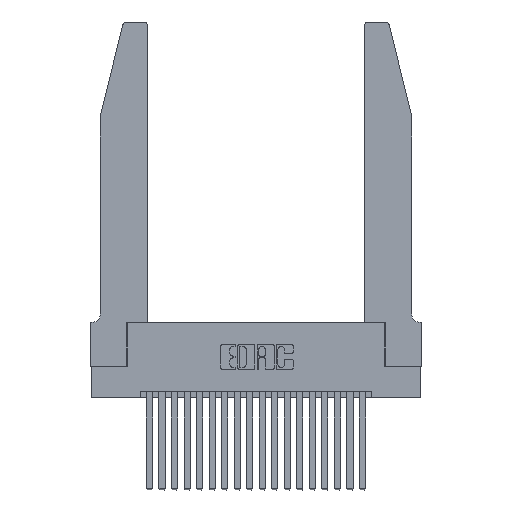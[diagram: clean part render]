
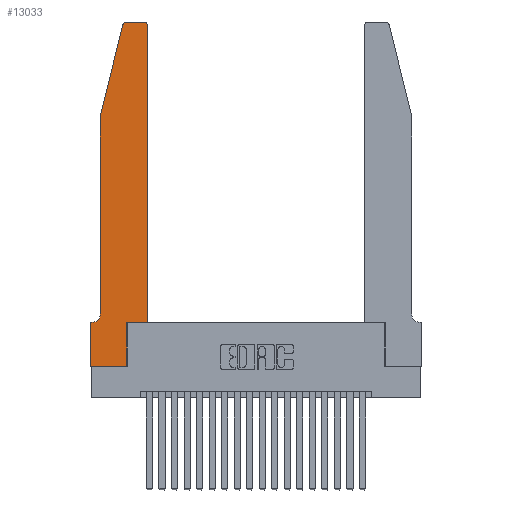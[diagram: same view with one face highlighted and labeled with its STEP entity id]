
A CAD part, top view. The second image highlights one B-rep face of the part: STEP entity #13033.
In plain terms, the highlighted planar face has unit normal (0, 0, 1).
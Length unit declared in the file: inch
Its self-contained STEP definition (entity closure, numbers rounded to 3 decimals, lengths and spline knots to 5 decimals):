
#79 = VERTEX_POINT ( 'NONE', #5755 ) ;
#144 = VERTEX_POINT ( 'NONE', #3099 ) ;
#146 = AXIS2_PLACEMENT_3D ( 'NONE', #11177, #937, #12860 ) ;
#159 = CARTESIAN_POINT ( 'NONE',  ( 0.0755, 2., 0.37 ) ) ;
#636 = EDGE_CURVE ( 'NONE', #144, #15574, #2656, .T. ) ;
#766 = CARTESIAN_POINT ( 'NONE',  ( 0.2865, 0.35, 0.37 ) ) ;
#859 = VECTOR ( 'NONE', #21269, 39.37008 ) ;
#937 = DIRECTION ( 'NONE',  ( 0., 0., -1. ) ) ;
#1041 = VERTEX_POINT ( 'NONE', #2652 ) ;
#1307 = EDGE_CURVE ( 'NONE', #15574, #6446, #21645, .T. ) ;
#1614 = CARTESIAN_POINT ( 'NONE',  ( 0.2605, 2.75, 0.37 ) ) ;
#1721 = CIRCLE ( 'NONE', #17137, 0.03 ) ;
#1864 = DIRECTION ( 'NONE',  ( -0.239, -0.971, 0. ) ) ;
#1951 = LINE ( 'NONE', #6266, #859 ) ;
#2418 = VECTOR ( 'NONE', #10659, 39.37008 ) ;
#2652 = CARTESIAN_POINT ( 'NONE',  ( 0.0755, 2., 0.37 ) ) ;
#2656 = LINE ( 'NONE', #14049, #6711 ) ;
#3094 = EDGE_CURVE ( 'NONE', #12554, #9892, #11370, .T. ) ;
#3099 = CARTESIAN_POINT ( 'NONE',  ( 0.0055, 0.35, 0.37 ) ) ;
#3180 = DIRECTION ( 'NONE',  ( 0., 1., 0. ) ) ;
#3273 = VERTEX_POINT ( 'NONE', #12145 ) ;
#3315 = CIRCLE ( 'NONE', #20019, 0.03 ) ;
#3813 = ORIENTED_EDGE ( 'NONE', *, *, #20375, .T. ) ;
#3968 = EDGE_CURVE ( 'NONE', #19969, #1041, #7945, .T. ) ;
#4036 = ORIENTED_EDGE ( 'NONE', *, *, #1307, .T. ) ;
#4055 = FACE_OUTER_BOUND ( 'NONE', #10293, .T. ) ;
#4132 = DIRECTION ( 'NONE',  ( -1., 0., 0. ) ) ;
#4140 = VERTEX_POINT ( 'NONE', #7461 ) ;
#4329 = ORIENTED_EDGE ( 'NONE', *, *, #5721, .T. ) ;
#4468 = EDGE_CURVE ( 'NONE', #13778, #19969, #3315, .T. ) ;
#4832 = PLANE ( 'NONE',  #12000 ) ;
#5020 = CARTESIAN_POINT ( 'NONE',  ( 0.284, 2.72, 0.37 ) ) ;
#5336 = CARTESIAN_POINT ( 'NONE',  ( 0.284, 2.75, 0.37 ) ) ;
#5721 = EDGE_CURVE ( 'NONE', #79, #144, #11518, .T. ) ;
#5755 = CARTESIAN_POINT ( 'NONE',  ( 0.0755, 0.42, 0.37 ) ) ;
#6121 = EDGE_CURVE ( 'NONE', #3273, #11683, #12017, .T. ) ;
#6266 = CARTESIAN_POINT ( 'NONE',  ( 0., 0., 0.37 ) ) ;
#6375 = VECTOR ( 'NONE', #3180, 39.37008 ) ;
#6446 = VERTEX_POINT ( 'NONE', #18388 ) ;
#6575 = CARTESIAN_POINT ( 'NONE',  ( 0.4505, 0.35, 0.37 ) ) ;
#6664 = CARTESIAN_POINT ( 'NONE',  ( 0.4505, 0.35, 0.37 ) ) ;
#6711 = VECTOR ( 'NONE', #4132, 39.37008 ) ;
#6764 = DIRECTION ( 'NONE',  ( 1., 0., 0. ) ) ;
#7377 = LINE ( 'NONE', #1614, #11829 ) ;
#7461 = CARTESIAN_POINT ( 'NONE',  ( 0.4205, 2.75, 0.37 ) ) ;
#7866 = CARTESIAN_POINT ( 'NONE',  ( 0.4505, 2.72, 0.37 ) ) ;
#7945 = LINE ( 'NONE', #159, #21787 ) ;
#8285 = DIRECTION ( 'NONE',  ( 0., 0., 1. ) ) ;
#8320 = VECTOR ( 'NONE', #9803, 39.37008 ) ;
#8470 = DIRECTION ( 'NONE',  ( -1., 0., 0. ) ) ;
#8974 = CARTESIAN_POINT ( 'NONE',  ( 0.0755, 2., 0.37 ) ) ;
#9081 = ORIENTED_EDGE ( 'NONE', *, *, #15283, .T. ) ;
#9416 = ORIENTED_EDGE ( 'NONE', *, *, #4468, .T. ) ;
#9509 = CARTESIAN_POINT ( 'NONE',  ( 0.4205, 2.72, 0.37 ) ) ;
#9803 = DIRECTION ( 'NONE',  ( 0., -1., 0. ) ) ;
#9892 = VERTEX_POINT ( 'NONE', #7866 ) ;
#9918 = CARTESIAN_POINT ( 'NONE',  ( 0., 0., 0.37 ) ) ;
#10293 = EDGE_LOOP ( 'NONE', ( #3813, #9416, #19080, #15966, #4329, #10685, #4036, #19844, #13311, #9081, #21375, #20774 ) ) ;
#10659 = DIRECTION ( 'NONE',  ( 0., -1., 0. ) ) ;
#10685 = ORIENTED_EDGE ( 'NONE', *, *, #636, .T. ) ;
#11177 = CARTESIAN_POINT ( 'NONE',  ( 0.0055, 0.42, 0.37 ) ) ;
#11202 = DIRECTION ( 'NONE',  ( 1., 0., 0. ) ) ;
#11370 = LINE ( 'NONE', #6664, #6375 ) ;
#11465 = LINE ( 'NONE', #8974, #2418 ) ;
#11518 = CIRCLE ( 'NONE', #146, 0.07 ) ;
#11683 = VERTEX_POINT ( 'NONE', #14509 ) ;
#11746 = EDGE_CURVE ( 'NONE', #6446, #3273, #1951, .T. ) ;
#11829 = VECTOR ( 'NONE', #8470, 39.37008 ) ;
#12000 = AXIS2_PLACEMENT_3D ( 'NONE', #18290, #8285, #19961 ) ;
#12017 = LINE ( 'NONE', #766, #20927 ) ;
#12027 = LINE ( 'NONE', #6575, #19879 ) ;
#12145 = CARTESIAN_POINT ( 'NONE',  ( 0.2865, 0., 0.37 ) ) ;
#12247 = CARTESIAN_POINT ( 'NONE',  ( 0.25487, 2.72718, 0.37 ) ) ;
#12554 = VERTEX_POINT ( 'NONE', #18672 ) ;
#12694 = DIRECTION ( 'NONE',  ( 0., 1., 0. ) ) ;
#12860 = DIRECTION ( 'NONE',  ( -1., 0., 0. ) ) ;
#13033 = ADVANCED_FACE ( 'NONE', ( #4055 ), #4832, .T. ) ;
#13311 = ORIENTED_EDGE ( 'NONE', *, *, #6121, .T. ) ;
#13778 = VERTEX_POINT ( 'NONE', #5336 ) ;
#14002 = CARTESIAN_POINT ( 'NONE',  ( 0., 0.35, 0.37 ) ) ;
#14049 = CARTESIAN_POINT ( 'NONE',  ( 0.0755, 0.35, 0.37 ) ) ;
#14509 = CARTESIAN_POINT ( 'NONE',  ( 0.2865, 0.35, 0.37 ) ) ;
#15283 = EDGE_CURVE ( 'NONE', #11683, #12554, #12027, .T. ) ;
#15574 = VERTEX_POINT ( 'NONE', #14002 ) ;
#15966 = ORIENTED_EDGE ( 'NONE', *, *, #16235, .T. ) ;
#16235 = EDGE_CURVE ( 'NONE', #1041, #79, #11465, .T. ) ;
#16710 = DIRECTION ( 'NONE',  ( 1., 0., 0. ) ) ;
#16808 = DIRECTION ( 'NONE',  ( 0., 0., 1. ) ) ;
#17137 = AXIS2_PLACEMENT_3D ( 'NONE', #9509, #21203, #11202 ) ;
#18290 = CARTESIAN_POINT ( 'NONE',  ( 0., 0.35, 0.37 ) ) ;
#18388 = CARTESIAN_POINT ( 'NONE',  ( 0., 0., 0.37 ) ) ;
#18672 = CARTESIAN_POINT ( 'NONE',  ( 0.4505, 0.35, 0.37 ) ) ;
#19080 = ORIENTED_EDGE ( 'NONE', *, *, #3968, .T. ) ;
#19529 = EDGE_CURVE ( 'NONE', #9892, #4140, #1721, .T. ) ;
#19844 = ORIENTED_EDGE ( 'NONE', *, *, #11746, .T. ) ;
#19879 = VECTOR ( 'NONE', #16710, 39.37008 ) ;
#19961 = DIRECTION ( 'NONE',  ( 1., 0., 0. ) ) ;
#19969 = VERTEX_POINT ( 'NONE', #12247 ) ;
#20019 = AXIS2_PLACEMENT_3D ( 'NONE', #5020, #16808, #6764 ) ;
#20375 = EDGE_CURVE ( 'NONE', #4140, #13778, #7377, .T. ) ;
#20774 = ORIENTED_EDGE ( 'NONE', *, *, #19529, .T. ) ;
#20927 = VECTOR ( 'NONE', #12694, 39.37008 ) ;
#21203 = DIRECTION ( 'NONE',  ( 0., 0., 1. ) ) ;
#21269 = DIRECTION ( 'NONE',  ( 1., 0., 0. ) ) ;
#21375 = ORIENTED_EDGE ( 'NONE', *, *, #3094, .T. ) ;
#21645 = LINE ( 'NONE', #9918, #8320 ) ;
#21787 = VECTOR ( 'NONE', #1864, 39.37008 ) ;
